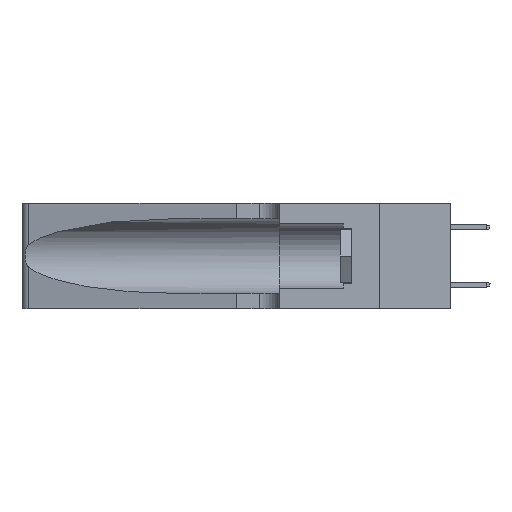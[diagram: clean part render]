
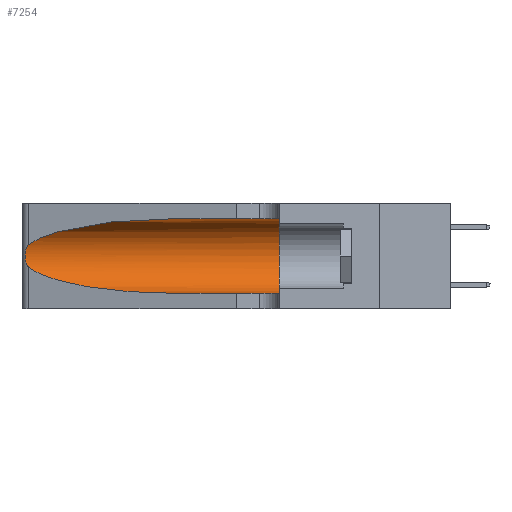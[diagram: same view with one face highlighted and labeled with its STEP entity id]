
A CAD part, left-side view. The second image highlights one B-rep face of the part: STEP entity #7254.
In plain terms, the highlighted cylindrical face has radius 3.308 mm (diameter 6.617 mm), a partial arc.
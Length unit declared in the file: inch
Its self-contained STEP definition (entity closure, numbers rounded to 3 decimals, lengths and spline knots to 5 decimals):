
#184 = CARTESIAN_POINT ( 'NONE',  ( 0.25487, 1.22718, 0.22369 ) ) ;
#316 = CARTESIAN_POINT ( 'NONE',  ( 0.26075, 1.23896, 0.178 ) ) ;
#752 = CARTESIAN_POINT ( 'NONE',  ( 0.18966, 0.96281, 0.05475 ) ) ;
#865 = VECTOR ( 'NONE', #4483, 39.37008 ) ;
#1611 = EDGE_CURVE ( 'NONE', #16743, #10099, #22901, .T. ) ;
#1933 = ORIENTED_EDGE ( 'NONE', *, *, #20501, .T. ) ;
#2436 = CARTESIAN_POINT ( 'NONE',  ( 0.25555, 1.22993, 0.14849 ) ) ;
#2576 = CARTESIAN_POINT ( 'NONE',  ( 0.26075, 1.23896, 0.19203 ) ) ;
#2729 = AXIS2_PLACEMENT_3D ( 'NONE', #25378, #22537, #3222 ) ;
#3178 = CARTESIAN_POINT ( 'NONE',  ( 0.18966, 0.96281, 0.31525 ) ) ;
#3195 = CIRCLE ( 'NONE', #2729, 0.13025 ) ;
#3222 = DIRECTION ( 'NONE',  ( 0., 0., 1. ) ) ;
#4483 = DIRECTION ( 'NONE',  ( 0., -1., 0. ) ) ;
#4713 = CARTESIAN_POINT ( 'NONE',  ( 0.25487, 1.22718, 0.14631 ) ) ;
#4848 = CARTESIAN_POINT ( 'NONE',  ( 0.25555, 1.22994, 0.2215 ) ) ;
#5007 = CARTESIAN_POINT ( 'NONE',  ( 0.1305, 0.72297, 0.05475 ) ) ;
#5354 =( BOUNDED_CURVE ( )  B_SPLINE_CURVE ( 3, ( #11547, #20227, #752, #5007 ),
 .UNSPECIFIED., .F., .T. ) 
 B_SPLINE_CURVE_WITH_KNOTS ( ( 4, 4 ),
 ( 3.44316, 4.71239 ),
 .UNSPECIFIED. ) 
 CURVE ( )  GEOMETRIC_REPRESENTATION_ITEM ( )  RATIONAL_B_SPLINE_CURVE ( ( 1., 0.87, 0.87, 1. ) ) 
 REPRESENTATION_ITEM ( '' )  );
#5871 = VERTEX_POINT ( 'NONE', #16546 ) ;
#6848 = CARTESIAN_POINT ( 'NONE',  ( 0.26017, 1.23833, 0.17102 ) ) ;
#7254 = ADVANCED_FACE ( 'NONE', ( #15736 ), #15874, .F. ) ;
#8251 = CARTESIAN_POINT ( 'NONE',  ( 0.1305, 0.35, 0.31525 ) ) ;
#8428 = ORIENTED_EDGE ( 'NONE', *, *, #1611, .F. ) ;
#8839 = EDGE_CURVE ( 'NONE', #23614, #9157, #9174, .T. ) ;
#8843 = CARTESIAN_POINT ( 'NONE',  ( 0.25639, 1.23184, 0.21858 ) ) ;
#9130 = VECTOR ( 'NONE', #19056, 39.37008 ) ;
#9157 = VERTEX_POINT ( 'NONE', #11160 ) ;
#9174 = LINE ( 'NONE', #17420, #865 ) ;
#9257 = CARTESIAN_POINT ( 'NONE',  ( 0.25639, 1.23186, 0.15144 ) ) ;
#9308 = EDGE_CURVE ( 'NONE', #16743, #5871, #10267, .T. ) ;
#10099 = VERTEX_POINT ( 'NONE', #8251 ) ;
#10267 =( BOUNDED_CURVE ( )  B_SPLINE_CURVE ( 3, ( #26625, #3178, #27054, #15967 ),
 .UNSPECIFIED., .F., .T. ) 
 B_SPLINE_CURVE_WITH_KNOTS ( ( 4, 4 ),
 ( 1.5708, 2.84003 ),
 .UNSPECIFIED. ) 
 CURVE ( )  GEOMETRIC_REPRESENTATION_ITEM ( )  RATIONAL_B_SPLINE_CURVE ( ( 1., 0.87, 0.87, 1. ) ) 
 REPRESENTATION_ITEM ( '' )  );
#11160 = CARTESIAN_POINT ( 'NONE',  ( 0.1305, 0.35, 0.05475 ) ) ;
#11235 = AXIS2_PLACEMENT_3D ( 'NONE', #20686, #27353, #16685 ) ;
#11547 = CARTESIAN_POINT ( 'NONE',  ( 0.25487, 1.22718, 0.14631 ) ) ;
#12120 = EDGE_CURVE ( 'NONE', #10099, #9157, #3195, .T. ) ;
#15241 = ORIENTED_EDGE ( 'NONE', *, *, #8839, .T. ) ;
#15641 = CARTESIAN_POINT ( 'NONE',  ( 0.26018, 1.23835, 0.19895 ) ) ;
#15736 = FACE_OUTER_BOUND ( 'NONE', #17676, .T. ) ;
#15874 = CYLINDRICAL_SURFACE ( 'NONE', #11235, 0.13025 ) ;
#15967 = CARTESIAN_POINT ( 'NONE',  ( 0.25487, 1.22718, 0.22369 ) ) ;
#16363 = CARTESIAN_POINT ( 'NONE',  ( 0.1305, 1.61858, 0.31525 ) ) ;
#16479 = CARTESIAN_POINT ( 'NONE',  ( 0.1305, 0.72297, 0.05475 ) ) ;
#16546 = CARTESIAN_POINT ( 'NONE',  ( 0.25487, 1.22718, 0.22369 ) ) ;
#16685 = DIRECTION ( 'NONE',  ( 0., 0., -1. ) ) ;
#16743 = VERTEX_POINT ( 'NONE', #24989 ) ;
#17235 = VERTEX_POINT ( 'NONE', #17976 ) ;
#17420 = CARTESIAN_POINT ( 'NONE',  ( 0.1305, 1.61858, 0.05475 ) ) ;
#17676 = EDGE_LOOP ( 'NONE', ( #19656, #1933, #24556, #15241, #19761, #8428 ) ) ;
#17923 = CARTESIAN_POINT ( 'NONE',  ( 0.25854, 1.2359, 0.20912 ) ) ;
#17976 = CARTESIAN_POINT ( 'NONE',  ( 0.25487, 1.22718, 0.14631 ) ) ;
#19056 = DIRECTION ( 'NONE',  ( 0., -1., 0. ) ) ;
#19656 = ORIENTED_EDGE ( 'NONE', *, *, #9308, .T. ) ;
#19740 = B_SPLINE_CURVE_WITH_KNOTS ( 'NONE', 3,
 ( #184, #4848, #8843, #26173, #17923, #15641, #2576, #316, #6848, #24176, #21912, #9257, #2436, #4713 ),
 .UNSPECIFIED., .F., .F.,
 ( 4, 2, 2, 2, 2, 2, 4 ),
 ( 0., 0.00027, 0.00053, 0.00107, 0.0016, 0.00187, 0.00214 ),
 .UNSPECIFIED. ) ;
#19761 = ORIENTED_EDGE ( 'NONE', *, *, #12120, .F. ) ;
#20227 = CARTESIAN_POINT ( 'NONE',  ( 0.2373, 1.15595, 0.08982 ) ) ;
#20501 = EDGE_CURVE ( 'NONE', #5871, #17235, #19740, .T. ) ;
#20686 = CARTESIAN_POINT ( 'NONE',  ( 0.1305, 1.61858, 0.185 ) ) ;
#21912 = CARTESIAN_POINT ( 'NONE',  ( 0.25789, 1.23486, 0.15765 ) ) ;
#22537 = DIRECTION ( 'NONE',  ( 0., 1., 0. ) ) ;
#22901 = LINE ( 'NONE', #16363, #9130 ) ;
#22939 = EDGE_CURVE ( 'NONE', #17235, #23614, #5354, .T. ) ;
#23614 = VERTEX_POINT ( 'NONE', #16479 ) ;
#24176 = CARTESIAN_POINT ( 'NONE',  ( 0.25856, 1.23593, 0.16098 ) ) ;
#24556 = ORIENTED_EDGE ( 'NONE', *, *, #22939, .T. ) ;
#24989 = CARTESIAN_POINT ( 'NONE',  ( 0.1305, 0.72297, 0.31525 ) ) ;
#25378 = CARTESIAN_POINT ( 'NONE',  ( 0.1305, 0.35, 0.185 ) ) ;
#26173 = CARTESIAN_POINT ( 'NONE',  ( 0.25787, 1.23484, 0.2124 ) ) ;
#26625 = CARTESIAN_POINT ( 'NONE',  ( 0.1305, 0.72297, 0.31525 ) ) ;
#27054 = CARTESIAN_POINT ( 'NONE',  ( 0.2373, 1.15595, 0.28018 ) ) ;
#27353 = DIRECTION ( 'NONE',  ( 0., -1., 0. ) ) ;
